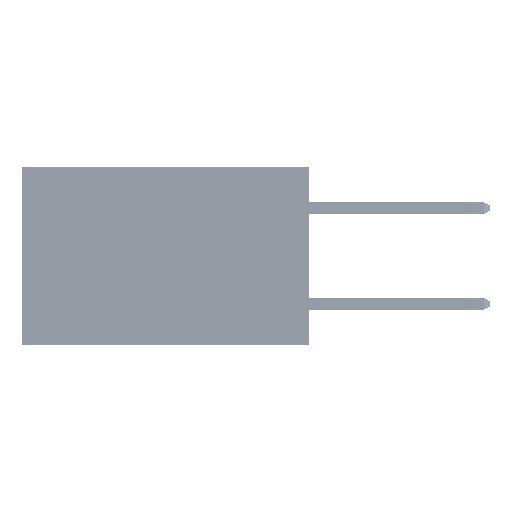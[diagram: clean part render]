
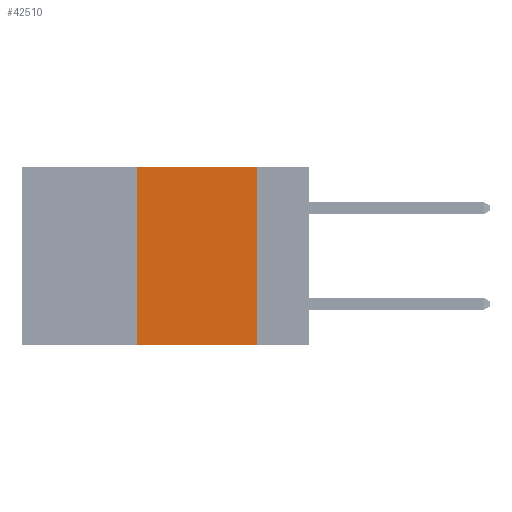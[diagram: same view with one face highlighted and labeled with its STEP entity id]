
A CAD part, left-side view. The second image highlights one B-rep face of the part: STEP entity #42510.
In plain terms, the highlighted planar face has unit normal (-1, 0, 0).
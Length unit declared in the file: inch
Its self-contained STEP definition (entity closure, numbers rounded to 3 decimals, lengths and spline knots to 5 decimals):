
#127 = VERTEX_POINT ( 'NONE', #29982 ) ;
#2163 = DIRECTION ( 'NONE',  ( 0., 0., 1. ) ) ;
#4173 = FACE_OUTER_BOUND ( 'NONE', #40837, .T. ) ;
#5141 = ORIENTED_EDGE ( 'NONE', *, *, #33161, .F. ) ;
#5209 = LINE ( 'NONE', #39235, #40704 ) ;
#6706 = EDGE_CURVE ( 'NONE', #127, #21980, #5209, .T. ) ;
#10567 = LINE ( 'NONE', #24072, #28020 ) ;
#11084 = VERTEX_POINT ( 'NONE', #38941 ) ;
#13126 = DIRECTION ( 'NONE',  ( 0., -1., 0. ) ) ;
#16694 = CARTESIAN_POINT ( 'NONE',  ( 0., 0.6, 0. ) ) ;
#17516 = VERTEX_POINT ( 'NONE', #23214 ) ;
#19211 = VECTOR ( 'NONE', #13126, 39.37008 ) ;
#21556 = DIRECTION ( 'NONE',  ( 1., 0., 0. ) ) ;
#21733 = PLANE ( 'NONE',  #33692 ) ;
#21887 = CARTESIAN_POINT ( 'NONE',  ( 0., 0.6, 0. ) ) ;
#21980 = VERTEX_POINT ( 'NONE', #36954 ) ;
#23214 = CARTESIAN_POINT ( 'NONE',  ( 0., 0.36, -0.37 ) ) ;
#24072 = CARTESIAN_POINT ( 'NONE',  ( 0., 0.6, -0.37 ) ) ;
#24946 = DIRECTION ( 'NONE',  ( 0., 0., -1. ) ) ;
#25160 = DIRECTION ( 'NONE',  ( 0., 0., -1. ) ) ;
#25513 = EDGE_CURVE ( 'NONE', #17516, #21980, #10567, .T. ) ;
#28020 = VECTOR ( 'NONE', #38524, 39.37008 ) ;
#29982 = CARTESIAN_POINT ( 'NONE',  ( 0., 0.11, 0. ) ) ;
#30943 = VECTOR ( 'NONE', #2163, 39.37008 ) ;
#31416 = LINE ( 'NONE', #16694, #19211 ) ;
#31969 = ORIENTED_EDGE ( 'NONE', *, *, #42426, .F. ) ;
#33161 = EDGE_CURVE ( 'NONE', #17516, #11084, #35014, .T. ) ;
#33217 = ORIENTED_EDGE ( 'NONE', *, *, #25513, .T. ) ;
#33692 = AXIS2_PLACEMENT_3D ( 'NONE', #21887, #21556, #25160 ) ;
#35014 = LINE ( 'NONE', #46657, #30943 ) ;
#36954 = CARTESIAN_POINT ( 'NONE',  ( 0., 0.11, -0.37 ) ) ;
#38524 = DIRECTION ( 'NONE',  ( 0., -1., 0. ) ) ;
#38681 = ORIENTED_EDGE ( 'NONE', *, *, #6706, .F. ) ;
#38941 = CARTESIAN_POINT ( 'NONE',  ( 0., 0.36, 0. ) ) ;
#39235 = CARTESIAN_POINT ( 'NONE',  ( 0., 0.11, 0. ) ) ;
#40704 = VECTOR ( 'NONE', #24946, 39.37008 ) ;
#40837 = EDGE_LOOP ( 'NONE', ( #38681, #31969, #5141, #33217 ) ) ;
#42426 = EDGE_CURVE ( 'NONE', #11084, #127, #31416, .T. ) ;
#42510 = ADVANCED_FACE ( 'NONE', ( #4173 ), #21733, .F. ) ;
#46657 = CARTESIAN_POINT ( 'NONE',  ( 0., 0.36, 0. ) ) ;
